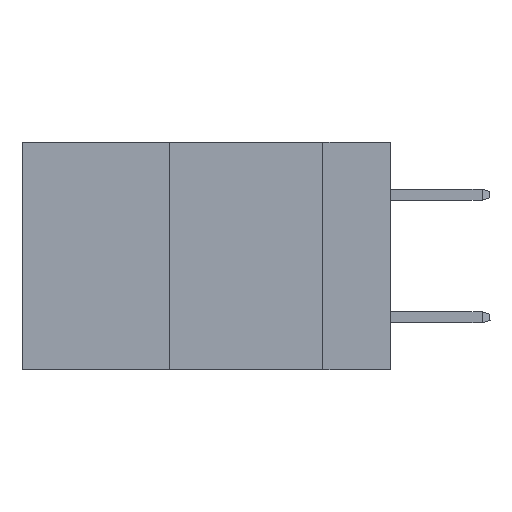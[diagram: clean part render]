
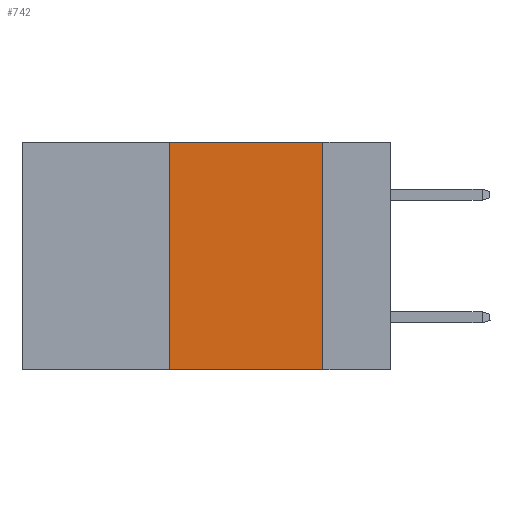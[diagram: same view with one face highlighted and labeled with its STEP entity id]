
A CAD part, left-side view. The second image highlights one B-rep face of the part: STEP entity #742.
In plain terms, the highlighted planar face has unit normal (-1, 0, 0).
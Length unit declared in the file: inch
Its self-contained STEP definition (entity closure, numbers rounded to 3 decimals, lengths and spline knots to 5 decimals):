
#177 = AXIS2_PLACEMENT_3D ( 'NONE', #5094, #7218, #12167 ) ;
#742 = ADVANCED_FACE ( 'NONE', ( #4069 ), #9174, .F. ) ;
#1179 = LINE ( 'NONE', #7382, #8801 ) ;
#1628 = EDGE_CURVE ( 'NONE', #10504, #9140, #2948, .T. ) ;
#2571 = LINE ( 'NONE', #6799, #3435 ) ;
#2703 = DIRECTION ( 'NONE',  ( 0., -1., 0. ) ) ;
#2948 = LINE ( 'NONE', #3899, #4920 ) ;
#3289 = ORIENTED_EDGE ( 'NONE', *, *, #1628, .F. ) ;
#3435 = VECTOR ( 'NONE', #2703, 39.37008 ) ;
#3899 = CARTESIAN_POINT ( 'NONE',  ( 0., 0.11, 0. ) ) ;
#4069 = FACE_OUTER_BOUND ( 'NONE', #13063, .T. ) ;
#4091 = VECTOR ( 'NONE', #11421, 39.37008 ) ;
#4131 = LINE ( 'NONE', #8291, #4091 ) ;
#4431 = CARTESIAN_POINT ( 'NONE',  ( 0., 0.36, 0. ) ) ;
#4920 = VECTOR ( 'NONE', #7114, 39.37008 ) ;
#5094 = CARTESIAN_POINT ( 'NONE',  ( 0., 0.6, 0. ) ) ;
#5737 = VERTEX_POINT ( 'NONE', #4431 ) ;
#5804 = ORIENTED_EDGE ( 'NONE', *, *, #7651, .T. ) ;
#6569 = CARTESIAN_POINT ( 'NONE',  ( 0., 0.11, -0.37 ) ) ;
#6799 = CARTESIAN_POINT ( 'NONE',  ( 0., 0.6, -0.37 ) ) ;
#7114 = DIRECTION ( 'NONE',  ( 0., 0., -1. ) ) ;
#7218 = DIRECTION ( 'NONE',  ( 1., 0., 0. ) ) ;
#7382 = CARTESIAN_POINT ( 'NONE',  ( 0., 0.36, 0. ) ) ;
#7651 = EDGE_CURVE ( 'NONE', #11191, #9140, #2571, .T. ) ;
#7892 = ORIENTED_EDGE ( 'NONE', *, *, #8037, .F. ) ;
#7992 = ORIENTED_EDGE ( 'NONE', *, *, #13050, .F. ) ;
#8037 = EDGE_CURVE ( 'NONE', #5737, #10504, #4131, .T. ) ;
#8291 = CARTESIAN_POINT ( 'NONE',  ( 0., 0.6, 0. ) ) ;
#8801 = VECTOR ( 'NONE', #9599, 39.37008 ) ;
#9140 = VERTEX_POINT ( 'NONE', #6569 ) ;
#9174 = PLANE ( 'NONE',  #177 ) ;
#9599 = DIRECTION ( 'NONE',  ( 0., 0., 1. ) ) ;
#10504 = VERTEX_POINT ( 'NONE', #13084 ) ;
#11191 = VERTEX_POINT ( 'NONE', #12389 ) ;
#11421 = DIRECTION ( 'NONE',  ( 0., -1., 0. ) ) ;
#12167 = DIRECTION ( 'NONE',  ( 0., 0., -1. ) ) ;
#12389 = CARTESIAN_POINT ( 'NONE',  ( 0., 0.36, -0.37 ) ) ;
#13050 = EDGE_CURVE ( 'NONE', #11191, #5737, #1179, .T. ) ;
#13063 = EDGE_LOOP ( 'NONE', ( #3289, #7892, #7992, #5804 ) ) ;
#13084 = CARTESIAN_POINT ( 'NONE',  ( 0., 0.11, 0. ) ) ;
